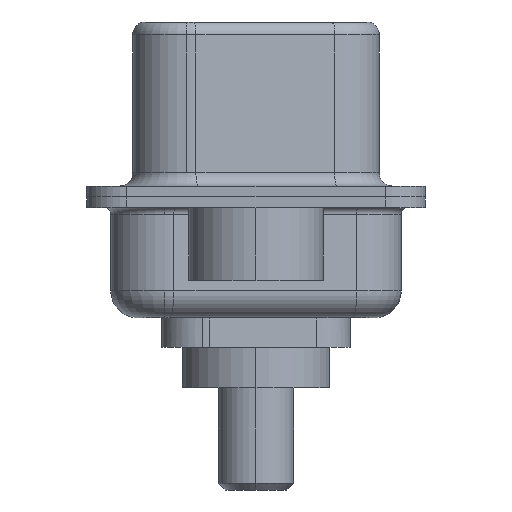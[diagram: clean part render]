
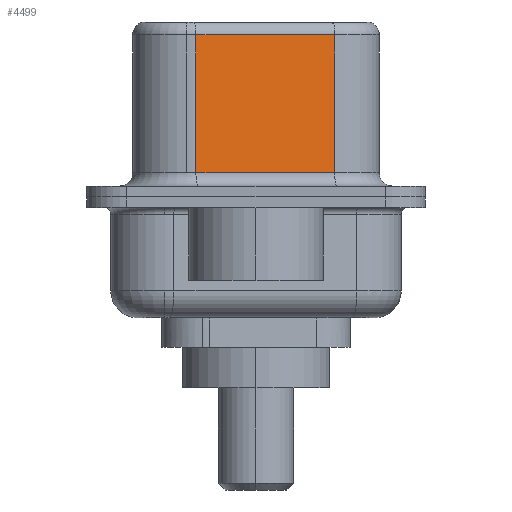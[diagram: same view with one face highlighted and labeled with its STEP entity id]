
A CAD part, left-side view. The second image highlights one B-rep face of the part: STEP entity #4499.
In plain terms, the highlighted planar face has unit normal (-0.985, -0.174, 0).
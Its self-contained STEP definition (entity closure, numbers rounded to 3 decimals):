
#1132 = CARTESIAN_POINT ( 'NONE',  ( 4.585, -2.927, 6.52 ) ) ;
#1349 = CARTESIAN_POINT ( 'NONE',  ( 3.675, 2.233, 6.02 ) ) ;
#1515 = LINE ( 'NONE', #4588, #13227 ) ;
#2744 = EDGE_CURVE ( 'NONE', #14082, #12154, #8868, .T. ) ;
#3373 = CARTESIAN_POINT ( 'NONE',  ( 4.585, -2.927, 6.52 ) ) ;
#3380 = DIRECTION ( 'NONE',  ( -0.174, 0.985, 0. ) ) ;
#3673 = EDGE_CURVE ( 'NONE', #5315, #5629, #4115, .T. ) ;
#4115 = LINE ( 'NONE', #4405, #12797 ) ;
#4285 = EDGE_CURVE ( 'NONE', #5629, #12154, #6790, .T. ) ;
#4405 = CARTESIAN_POINT ( 'NONE',  ( 3.675, 2.233, 6.52 ) ) ;
#4499 = ADVANCED_FACE ( 'NONE', ( #9585 ), #9054, .F. ) ;
#4581 = ORIENTED_EDGE ( 'NONE', *, *, #9113, .T. ) ;
#4588 = CARTESIAN_POINT ( 'NONE',  ( 4.585, -2.927, 6.02 ) ) ;
#4759 = DIRECTION ( 'NONE',  ( 0., 0., -1. ) ) ;
#5315 = VERTEX_POINT ( 'NONE', #1349 ) ;
#5374 = EDGE_LOOP ( 'NONE', ( #13738, #4581, #9611, #9115 ) ) ;
#5629 = VERTEX_POINT ( 'NONE', #7533 ) ;
#5755 = CARTESIAN_POINT ( 'NONE',  ( 4.585, -2.927, 0.9 ) ) ;
#6790 = LINE ( 'NONE', #5755, #9413 ) ;
#6906 = DIRECTION ( 'NONE',  ( 0.174, -0.985, 0. ) ) ;
#7533 = CARTESIAN_POINT ( 'NONE',  ( 3.675, 2.233, 0.9 ) ) ;
#7910 = DIRECTION ( 'NONE',  ( 0., 0., -1. ) ) ;
#8868 = LINE ( 'NONE', #3373, #11511 ) ;
#9054 = PLANE ( 'NONE',  #10008 ) ;
#9113 = EDGE_CURVE ( 'NONE', #14082, #5315, #1515, .T. ) ;
#9115 = ORIENTED_EDGE ( 'NONE', *, *, #4285, .T. ) ;
#9143 = DIRECTION ( 'NONE',  ( -0.174, 0.985, 0. ) ) ;
#9413 = VECTOR ( 'NONE', #6906, 1000. ) ;
#9417 = CARTESIAN_POINT ( 'NONE',  ( 4.585, -2.927, 6.02 ) ) ;
#9585 = FACE_OUTER_BOUND ( 'NONE', #5374, .T. ) ;
#9611 = ORIENTED_EDGE ( 'NONE', *, *, #3673, .T. ) ;
#10008 = AXIS2_PLACEMENT_3D ( 'NONE', #1132, #10187, #3380 ) ;
#10187 = DIRECTION ( 'NONE',  ( 0.985, 0.174, 0. ) ) ;
#11258 = CARTESIAN_POINT ( 'NONE',  ( 4.585, -2.927, 0.9 ) ) ;
#11511 = VECTOR ( 'NONE', #7910, 1000. ) ;
#12154 = VERTEX_POINT ( 'NONE', #11258 ) ;
#12797 = VECTOR ( 'NONE', #4759, 1000. ) ;
#13227 = VECTOR ( 'NONE', #9143, 1000. ) ;
#13738 = ORIENTED_EDGE ( 'NONE', *, *, #2744, .F. ) ;
#14082 = VERTEX_POINT ( 'NONE', #9417 ) ;
